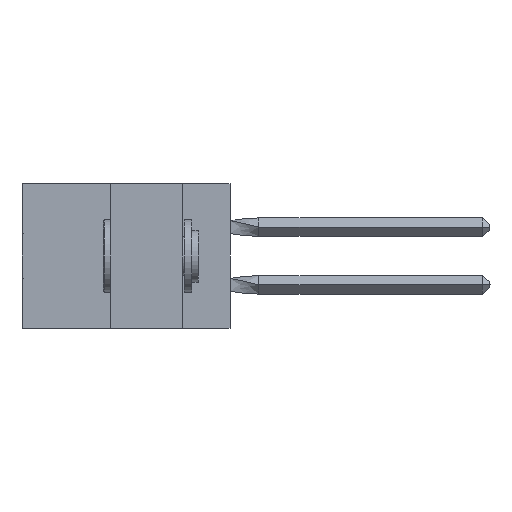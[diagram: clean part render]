
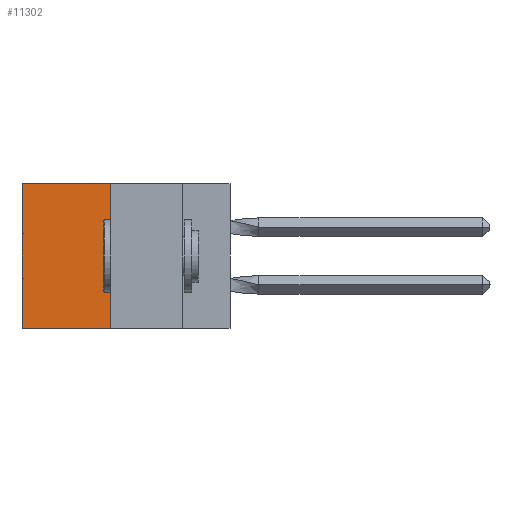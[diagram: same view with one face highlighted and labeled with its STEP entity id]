
A CAD part, left-side view. The second image highlights one B-rep face of the part: STEP entity #11302.
In plain terms, the highlighted planar face has unit normal (-1, 0, 0).
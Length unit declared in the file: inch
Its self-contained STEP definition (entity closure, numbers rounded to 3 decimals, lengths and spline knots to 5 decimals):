
#946 = CARTESIAN_POINT ( 'NONE',  ( 0.305, 0.413, -0.5 ) ) ;
#2783 = FACE_OUTER_BOUND ( 'NONE', #31734, .T. ) ;
#3443 = LINE ( 'NONE', #39970, #22637 ) ;
#3718 = DIRECTION ( 'NONE',  ( 0., 0., -1. ) ) ;
#3921 = DIRECTION ( 'NONE',  ( 0., 1., 0. ) ) ;
#3997 = DIRECTION ( 'NONE',  ( 0., 0., -1. ) ) ;
#5488 = VERTEX_POINT ( 'NONE', #37115 ) ;
#5774 = CARTESIAN_POINT ( 'NONE',  ( 0.305, 0.413, -0.5 ) ) ;
#6123 = CARTESIAN_POINT ( 'NONE',  ( 0.305, 0.72, -0.5 ) ) ;
#6378 = DIRECTION ( 'NONE',  ( 1., 0., 0. ) ) ;
#6955 = LINE ( 'NONE', #24942, #25576 ) ;
#8251 = DIRECTION ( 'NONE',  ( 0., 1., 0. ) ) ;
#9319 = EDGE_CURVE ( 'NONE', #23957, #35444, #32137, .T. ) ;
#11302 = ADVANCED_FACE ( 'NONE', ( #2783 ), #32536, .F. ) ;
#12746 = VECTOR ( 'NONE', #8251, 39.37008 ) ;
#14892 = LINE ( 'NONE', #22348, #12746 ) ;
#16058 = CARTESIAN_POINT ( 'NONE',  ( 0.305, 0.413, -0.5 ) ) ;
#17137 = ORIENTED_EDGE ( 'NONE', *, *, #27262, .T. ) ;
#18803 = DIRECTION ( 'NONE',  ( 0., 0., -1. ) ) ;
#19790 = ORIENTED_EDGE ( 'NONE', *, *, #29026, .T. ) ;
#21456 = AXIS2_PLACEMENT_3D ( 'NONE', #5774, #6378, #3997 ) ;
#21581 = CARTESIAN_POINT ( 'NONE',  ( 0.305, 0.413, 0. ) ) ;
#22348 = CARTESIAN_POINT ( 'NONE',  ( 0.305, 0.413, -0.5 ) ) ;
#22637 = VECTOR ( 'NONE', #18803, 39.37008 ) ;
#23957 = VERTEX_POINT ( 'NONE', #21581 ) ;
#24448 = ORIENTED_EDGE ( 'NONE', *, *, #42023, .F. ) ;
#24942 = CARTESIAN_POINT ( 'NONE',  ( 0.305, 0.413, 0. ) ) ;
#25576 = VECTOR ( 'NONE', #3921, 39.37008 ) ;
#27262 = EDGE_CURVE ( 'NONE', #23957, #5488, #6955, .T. ) ;
#29026 = EDGE_CURVE ( 'NONE', #5488, #40571, #3443, .T. ) ;
#31734 = EDGE_LOOP ( 'NONE', ( #19790, #24448, #41535, #17137 ) ) ;
#32137 = LINE ( 'NONE', #946, #45440 ) ;
#32536 = PLANE ( 'NONE',  #21456 ) ;
#35444 = VERTEX_POINT ( 'NONE', #16058 ) ;
#37115 = CARTESIAN_POINT ( 'NONE',  ( 0.305, 0.72, 0. ) ) ;
#39970 = CARTESIAN_POINT ( 'NONE',  ( 0.305, 0.72, -0.5 ) ) ;
#40571 = VERTEX_POINT ( 'NONE', #6123 ) ;
#41535 = ORIENTED_EDGE ( 'NONE', *, *, #9319, .F. ) ;
#42023 = EDGE_CURVE ( 'NONE', #35444, #40571, #14892, .T. ) ;
#45440 = VECTOR ( 'NONE', #3718, 39.37008 ) ;
